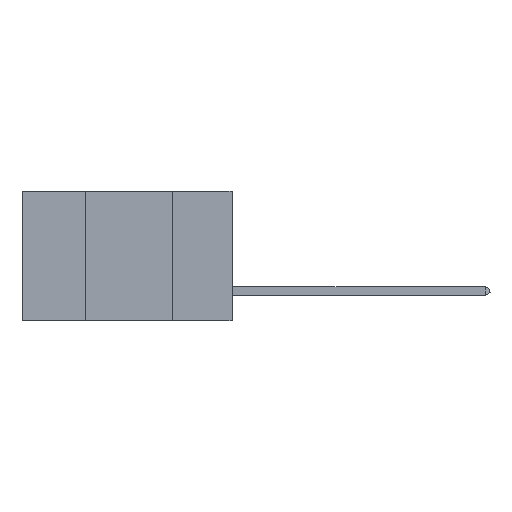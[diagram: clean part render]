
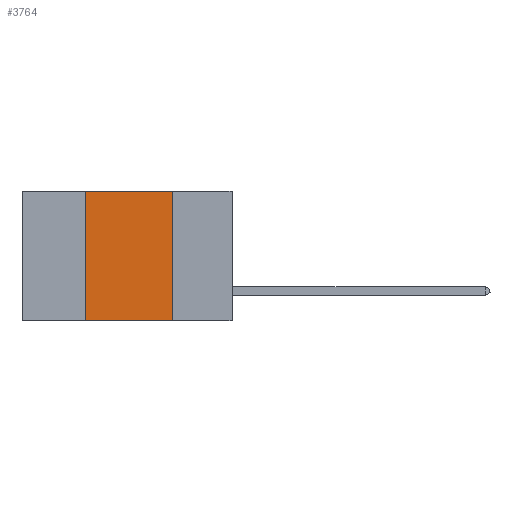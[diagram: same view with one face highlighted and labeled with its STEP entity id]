
A CAD part, left-side view. The second image highlights one B-rep face of the part: STEP entity #3764.
In plain terms, the highlighted planar face has unit normal (-1, 0, 0).
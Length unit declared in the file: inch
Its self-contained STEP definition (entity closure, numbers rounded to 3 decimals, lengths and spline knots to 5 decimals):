
#112 = EDGE_LOOP ( 'NONE', ( #3930, #4338, #12005, #7443 ) ) ;
#1752 = DIRECTION ( 'NONE',  ( 0., 0., -1. ) ) ;
#2011 = VECTOR ( 'NONE', #1752, 39.37008 ) ;
#2012 = DIRECTION ( 'NONE',  ( 1., 0., 0. ) ) ;
#2287 = LINE ( 'NONE', #10902, #14081 ) ;
#2875 = VERTEX_POINT ( 'NONE', #9542 ) ;
#3530 = VERTEX_POINT ( 'NONE', #9009 ) ;
#3764 = ADVANCED_FACE ( 'NONE', ( #10707 ), #10701, .F. ) ;
#3930 = ORIENTED_EDGE ( 'NONE', *, *, #6299, .F. ) ;
#4335 = VECTOR ( 'NONE', #16039, 39.37008 ) ;
#4338 = ORIENTED_EDGE ( 'NONE', *, *, #10865, .F. ) ;
#4460 = VERTEX_POINT ( 'NONE', #4789 ) ;
#4789 = CARTESIAN_POINT ( 'NONE',  ( 0., 0.17, -0.37 ) ) ;
#5728 = VECTOR ( 'NONE', #12741, 39.37008 ) ;
#5912 = DIRECTION ( 'NONE',  ( 0., 0., 1. ) ) ;
#6270 = EDGE_CURVE ( 'NONE', #8922, #4460, #6859, .T. ) ;
#6299 = EDGE_CURVE ( 'NONE', #3530, #4460, #8625, .T. ) ;
#6859 = LINE ( 'NONE', #15082, #5728 ) ;
#7007 = CARTESIAN_POINT ( 'NONE',  ( 0., 0.42, -0.37 ) ) ;
#7443 = ORIENTED_EDGE ( 'NONE', *, *, #6270, .T. ) ;
#7456 = CARTESIAN_POINT ( 'NONE',  ( 0., 0.6, 0. ) ) ;
#8625 = LINE ( 'NONE', #15342, #2011 ) ;
#8922 = VERTEX_POINT ( 'NONE', #7007 ) ;
#9009 = CARTESIAN_POINT ( 'NONE',  ( 0., 0.17, 0. ) ) ;
#9376 = EDGE_CURVE ( 'NONE', #8922, #2875, #2287, .T. ) ;
#9464 = DIRECTION ( 'NONE',  ( 0., 0., -1. ) ) ;
#9542 = CARTESIAN_POINT ( 'NONE',  ( 0., 0.42, 0. ) ) ;
#10615 = AXIS2_PLACEMENT_3D ( 'NONE', #15644, #2012, #9464 ) ;
#10701 = PLANE ( 'NONE',  #10615 ) ;
#10707 = FACE_OUTER_BOUND ( 'NONE', #112, .T. ) ;
#10865 = EDGE_CURVE ( 'NONE', #2875, #3530, #11832, .T. ) ;
#10902 = CARTESIAN_POINT ( 'NONE',  ( 0., 0.42, 0. ) ) ;
#11832 = LINE ( 'NONE', #7456, #4335 ) ;
#12005 = ORIENTED_EDGE ( 'NONE', *, *, #9376, .F. ) ;
#12741 = DIRECTION ( 'NONE',  ( 0., -1., 0. ) ) ;
#14081 = VECTOR ( 'NONE', #5912, 39.37008 ) ;
#15082 = CARTESIAN_POINT ( 'NONE',  ( 0., 0.6, -0.37 ) ) ;
#15342 = CARTESIAN_POINT ( 'NONE',  ( 0., 0.17, 0. ) ) ;
#15644 = CARTESIAN_POINT ( 'NONE',  ( 0., 0.6, 0. ) ) ;
#16039 = DIRECTION ( 'NONE',  ( 0., -1., 0. ) ) ;
